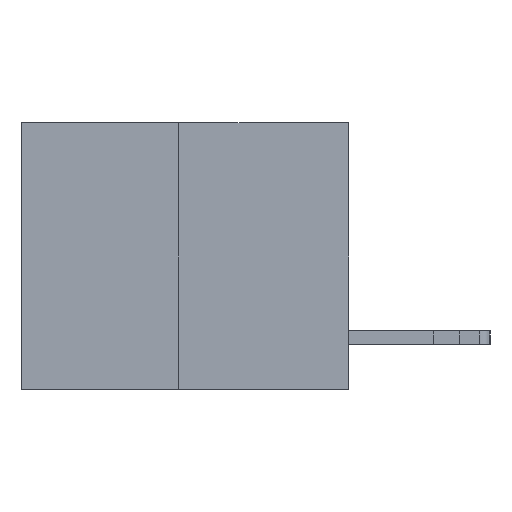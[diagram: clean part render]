
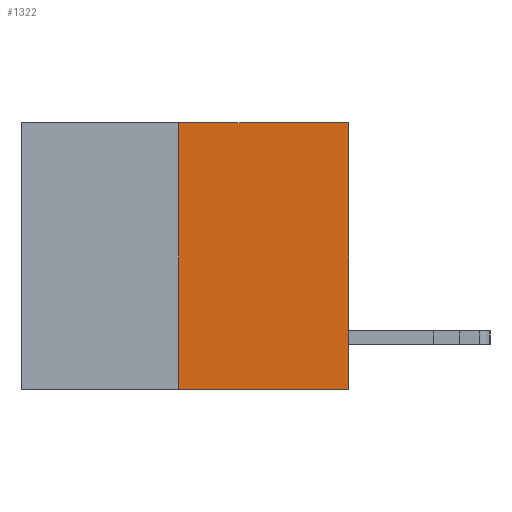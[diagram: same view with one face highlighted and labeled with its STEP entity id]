
A CAD part, left-side view. The second image highlights one B-rep face of the part: STEP entity #1322.
In plain terms, the highlighted planar face has unit normal (-1, 0, 0).
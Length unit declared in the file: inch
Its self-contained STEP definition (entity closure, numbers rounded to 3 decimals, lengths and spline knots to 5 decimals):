
#367 = VERTEX_POINT ( 'NONE', #3745 ) ;
#832 = VERTEX_POINT ( 'NONE', #22544 ) ;
#1052 = AXIS2_PLACEMENT_3D ( 'NONE', #20127, #18096, #1055 ) ;
#1055 = DIRECTION ( 'NONE',  ( 0., 0., -1. ) ) ;
#1322 = ADVANCED_FACE ( 'NONE', ( #12815 ), #19940, .F. ) ;
#1710 = CARTESIAN_POINT ( 'NONE',  ( 0., 0., -0.49 ) ) ;
#3617 = VECTOR ( 'NONE', #16029, 39.37008 ) ;
#3745 = CARTESIAN_POINT ( 'NONE',  ( 0., 0., 0. ) ) ;
#4540 = LINE ( 'NONE', #18422, #5865 ) ;
#5148 = DIRECTION ( 'NONE',  ( 0., 0., 1. ) ) ;
#5821 = EDGE_CURVE ( 'NONE', #832, #9413, #20606, .T. ) ;
#5865 = VECTOR ( 'NONE', #22678, 39.37008 ) ;
#7464 = VERTEX_POINT ( 'NONE', #1710 ) ;
#7830 = EDGE_CURVE ( 'NONE', #7464, #367, #24790, .T. ) ;
#8445 = CARTESIAN_POINT ( 'NONE',  ( 0., 0.312, -0.49 ) ) ;
#8864 = ORIENTED_EDGE ( 'NONE', *, *, #5821, .F. ) ;
#9413 = VERTEX_POINT ( 'NONE', #17701 ) ;
#9504 = EDGE_CURVE ( 'NONE', #832, #7464, #13500, .T. ) ;
#10369 = DIRECTION ( 'NONE',  ( 0., 0., 1. ) ) ;
#10714 = EDGE_CURVE ( 'NONE', #9413, #367, #4540, .T. ) ;
#12639 = ORIENTED_EDGE ( 'NONE', *, *, #10714, .F. ) ;
#12815 = FACE_OUTER_BOUND ( 'NONE', #21466, .T. ) ;
#13500 = LINE ( 'NONE', #13754, #3617 ) ;
#13616 = ORIENTED_EDGE ( 'NONE', *, *, #7830, .T. ) ;
#13754 = CARTESIAN_POINT ( 'NONE',  ( 0., 0.6, -0.49 ) ) ;
#15342 = CARTESIAN_POINT ( 'NONE',  ( 0., 0., 0. ) ) ;
#16029 = DIRECTION ( 'NONE',  ( 0., -1., 0. ) ) ;
#16651 = VECTOR ( 'NONE', #10369, 39.37008 ) ;
#17549 = VECTOR ( 'NONE', #5148, 39.37008 ) ;
#17701 = CARTESIAN_POINT ( 'NONE',  ( 0., 0.312, 0. ) ) ;
#18096 = DIRECTION ( 'NONE',  ( 1., 0., 0. ) ) ;
#18422 = CARTESIAN_POINT ( 'NONE',  ( 0., 0.6, 0. ) ) ;
#19940 = PLANE ( 'NONE',  #1052 ) ;
#20127 = CARTESIAN_POINT ( 'NONE',  ( 0., 0.6, 0. ) ) ;
#20606 = LINE ( 'NONE', #8445, #16651 ) ;
#21466 = EDGE_LOOP ( 'NONE', ( #8864, #22386, #13616, #12639 ) ) ;
#22386 = ORIENTED_EDGE ( 'NONE', *, *, #9504, .T. ) ;
#22544 = CARTESIAN_POINT ( 'NONE',  ( 0., 0.312, -0.49 ) ) ;
#22678 = DIRECTION ( 'NONE',  ( 0., -1., 0. ) ) ;
#24790 = LINE ( 'NONE', #15342, #17549 ) ;
